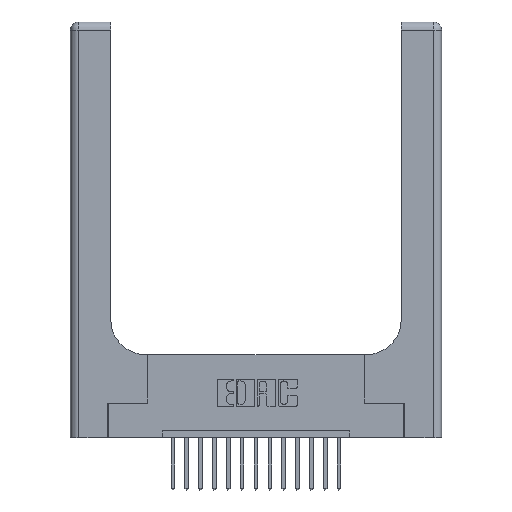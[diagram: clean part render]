
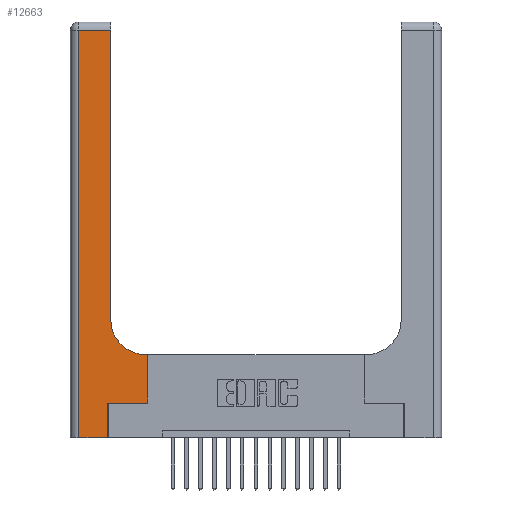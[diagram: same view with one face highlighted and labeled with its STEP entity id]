
A CAD part, top view. The second image highlights one B-rep face of the part: STEP entity #12663.
In plain terms, the highlighted planar face has unit normal (0, 0, 1).
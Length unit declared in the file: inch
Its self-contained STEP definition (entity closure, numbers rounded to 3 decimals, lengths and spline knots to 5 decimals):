
#578 = CARTESIAN_POINT ( 'NONE',  ( 0.2915, 2.94, 0.37 ) ) ;
#897 = CARTESIAN_POINT ( 'NONE',  ( 0.5415, 0.85, 0.37 ) ) ;
#961 = EDGE_CURVE ( 'NONE', #18680, #16068, #6552, .T. ) ;
#1081 = VECTOR ( 'NONE', #15306, 39.37008 ) ;
#1317 = ORIENTED_EDGE ( 'NONE', *, *, #12721, .T. ) ;
#1318 = LINE ( 'NONE', #12534, #1081 ) ;
#1417 = EDGE_CURVE ( 'NONE', #15546, #11579, #16151, .T. ) ;
#1517 = CARTESIAN_POINT ( 'NONE',  ( 0.06, 0., 0.37 ) ) ;
#1838 = ORIENTED_EDGE ( 'NONE', *, *, #18549, .T. ) ;
#1957 = DIRECTION ( 'NONE',  ( 0., 1., 0. ) ) ;
#2437 = LINE ( 'NONE', #11121, #12737 ) ;
#2473 = CARTESIAN_POINT ( 'NONE',  ( 0.2915, 0.85, 0.37 ) ) ;
#2675 = LINE ( 'NONE', #15426, #4513 ) ;
#3605 = EDGE_CURVE ( 'NONE', #14464, #18219, #7637, .T. ) ;
#3717 = DIRECTION ( 'NONE',  ( 0., 1., 0. ) ) ;
#3766 = VECTOR ( 'NONE', #6133, 39.37008 ) ;
#3820 = EDGE_CURVE ( 'NONE', #3866, #18680, #11992, .T. ) ;
#3866 = VERTEX_POINT ( 'NONE', #6831 ) ;
#4035 = DIRECTION ( 'NONE',  ( 1., 0., 0. ) ) ;
#4063 = FACE_OUTER_BOUND ( 'NONE', #11630, .T. ) ;
#4148 = ORIENTED_EDGE ( 'NONE', *, *, #961, .T. ) ;
#4180 = ORIENTED_EDGE ( 'NONE', *, *, #3820, .T. ) ;
#4513 = VECTOR ( 'NONE', #3717, 39.37008 ) ;
#4724 = AXIS2_PLACEMENT_3D ( 'NONE', #17759, #4829, #9103 ) ;
#4766 = PLANE ( 'NONE',  #4724 ) ;
#4770 = CARTESIAN_POINT ( 'NONE',  ( 0.5585, 0.6, 0.37 ) ) ;
#4829 = DIRECTION ( 'NONE',  ( 0., 0., -1. ) ) ;
#5038 = EDGE_CURVE ( 'NONE', #18219, #14297, #5320, .T. ) ;
#5320 = LINE ( 'NONE', #10664, #6438 ) ;
#6133 = DIRECTION ( 'NONE',  ( 1., 0., 0. ) ) ;
#6438 = VECTOR ( 'NONE', #1957, 39.37008 ) ;
#6552 = LINE ( 'NONE', #11271, #12321 ) ;
#6765 = DIRECTION ( 'NONE',  ( 0., 0., -1. ) ) ;
#6831 = CARTESIAN_POINT ( 'NONE',  ( 0.5415, 0.6, 0.37 ) ) ;
#6853 = CARTESIAN_POINT ( 'NONE',  ( 0.269, 0.25, 0.37 ) ) ;
#7637 = LINE ( 'NONE', #6853, #3766 ) ;
#7930 = LINE ( 'NONE', #8340, #15452 ) ;
#8210 = DIRECTION ( 'NONE',  ( -1., 0., 0. ) ) ;
#8288 = DIRECTION ( 'NONE',  ( -1., 0., 0. ) ) ;
#8340 = CARTESIAN_POINT ( 'NONE',  ( 0.2915, 0.6, 0.37 ) ) ;
#8379 = DIRECTION ( 'NONE',  ( 0., 1., 0. ) ) ;
#8787 = EDGE_CURVE ( 'NONE', #16068, #15546, #2437, .T. ) ;
#9103 = DIRECTION ( 'NONE',  ( -1., 0., 0. ) ) ;
#10664 = CARTESIAN_POINT ( 'NONE',  ( 0.5585, 0.25, 0.37 ) ) ;
#10905 = CARTESIAN_POINT ( 'NONE',  ( 0.269, 0.25, 0.37 ) ) ;
#11121 = CARTESIAN_POINT ( 'NONE',  ( 0., 2.94, 0.37 ) ) ;
#11271 = CARTESIAN_POINT ( 'NONE',  ( 0.2915, 3., 0.37 ) ) ;
#11579 = VERTEX_POINT ( 'NONE', #1517 ) ;
#11598 = CARTESIAN_POINT ( 'NONE',  ( 0.5585, 0.25, 0.37 ) ) ;
#11630 = EDGE_LOOP ( 'NONE', ( #4148, #14099, #13264, #1838, #13771, #11664, #17507, #1317, #4180 ) ) ;
#11664 = ORIENTED_EDGE ( 'NONE', *, *, #3605, .T. ) ;
#11992 = CIRCLE ( 'NONE', #16986, 0.25 ) ;
#12238 = CARTESIAN_POINT ( 'NONE',  ( 0.269, 0., 0.37 ) ) ;
#12270 = EDGE_CURVE ( 'NONE', #13856, #14464, #2675, .T. ) ;
#12321 = VECTOR ( 'NONE', #8379, 39.37008 ) ;
#12323 = VECTOR ( 'NONE', #14132, 39.37008 ) ;
#12534 = CARTESIAN_POINT ( 'NONE',  ( 0., 0., 0.37 ) ) ;
#12663 = ADVANCED_FACE ( 'NONE', ( #4063 ), #4766, .F. ) ;
#12721 = EDGE_CURVE ( 'NONE', #14297, #3866, #7930, .T. ) ;
#12737 = VECTOR ( 'NONE', #8288, 39.37008 ) ;
#13264 = ORIENTED_EDGE ( 'NONE', *, *, #1417, .T. ) ;
#13771 = ORIENTED_EDGE ( 'NONE', *, *, #12270, .T. ) ;
#13856 = VERTEX_POINT ( 'NONE', #12238 ) ;
#14099 = ORIENTED_EDGE ( 'NONE', *, *, #8787, .T. ) ;
#14132 = DIRECTION ( 'NONE',  ( 0., -1., 0. ) ) ;
#14297 = VERTEX_POINT ( 'NONE', #4770 ) ;
#14464 = VERTEX_POINT ( 'NONE', #10905 ) ;
#15306 = DIRECTION ( 'NONE',  ( 1., 0., 0. ) ) ;
#15426 = CARTESIAN_POINT ( 'NONE',  ( 0.269, 0., 0.37 ) ) ;
#15452 = VECTOR ( 'NONE', #8210, 39.37008 ) ;
#15546 = VERTEX_POINT ( 'NONE', #16918 ) ;
#16068 = VERTEX_POINT ( 'NONE', #578 ) ;
#16151 = LINE ( 'NONE', #16591, #12323 ) ;
#16591 = CARTESIAN_POINT ( 'NONE',  ( 0.06, 3., 0.37 ) ) ;
#16918 = CARTESIAN_POINT ( 'NONE',  ( 0.06, 2.94, 0.37 ) ) ;
#16986 = AXIS2_PLACEMENT_3D ( 'NONE', #897, #6765, #4035 ) ;
#17507 = ORIENTED_EDGE ( 'NONE', *, *, #5038, .T. ) ;
#17759 = CARTESIAN_POINT ( 'NONE',  ( 0., 3., 0.37 ) ) ;
#18219 = VERTEX_POINT ( 'NONE', #11598 ) ;
#18549 = EDGE_CURVE ( 'NONE', #11579, #13856, #1318, .T. ) ;
#18680 = VERTEX_POINT ( 'NONE', #2473 ) ;
